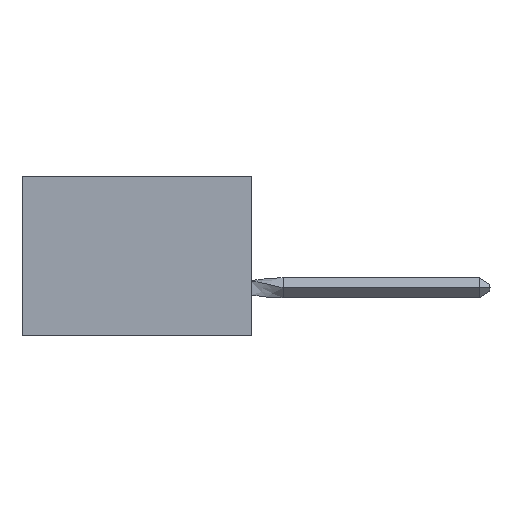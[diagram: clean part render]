
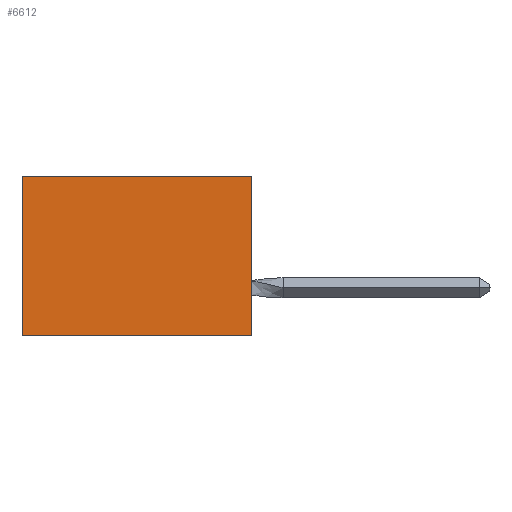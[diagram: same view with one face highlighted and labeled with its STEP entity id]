
A CAD part, left-side view. The second image highlights one B-rep face of the part: STEP entity #6612.
In plain terms, the highlighted planar face has unit normal (-1, 0, 0).
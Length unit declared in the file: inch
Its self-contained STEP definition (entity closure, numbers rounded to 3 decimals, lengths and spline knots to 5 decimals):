
#203 = VECTOR ( 'NONE', #4181, 39.37008 ) ;
#542 = PLANE ( 'NONE',  #6799 ) ;
#1179 = VECTOR ( 'NONE', #8908, 39.37008 ) ;
#1375 = EDGE_LOOP ( 'NONE', ( #3609, #6188, #13328, #8357 ) ) ;
#1581 = CARTESIAN_POINT ( 'NONE',  ( 0.305, 0., -0.5 ) ) ;
#2158 = VERTEX_POINT ( 'NONE', #9919 ) ;
#2236 = VECTOR ( 'NONE', #9385, 39.37008 ) ;
#2785 = LINE ( 'NONE', #3702, #1179 ) ;
#2906 = LINE ( 'NONE', #4169, #2236 ) ;
#3089 = EDGE_CURVE ( 'NONE', #11023, #5474, #4993, .T. ) ;
#3609 = ORIENTED_EDGE ( 'NONE', *, *, #3977, .T. ) ;
#3682 = VECTOR ( 'NONE', #5575, 39.37008 ) ;
#3702 = CARTESIAN_POINT ( 'NONE',  ( 0.305, 0., 0. ) ) ;
#3977 = EDGE_CURVE ( 'NONE', #4420, #5474, #2906, .T. ) ;
#4169 = CARTESIAN_POINT ( 'NONE',  ( 0.305, 0.72, -0.5 ) ) ;
#4181 = DIRECTION ( 'NONE',  ( 0., 0., -1. ) ) ;
#4420 = VERTEX_POINT ( 'NONE', #10097 ) ;
#4819 = CARTESIAN_POINT ( 'NONE',  ( 0.305, 0., -0.5 ) ) ;
#4993 = LINE ( 'NONE', #10900, #3682 ) ;
#5042 = LINE ( 'NONE', #6329, #203 ) ;
#5474 = VERTEX_POINT ( 'NONE', #9272 ) ;
#5575 = DIRECTION ( 'NONE',  ( 0., 1., 0. ) ) ;
#6188 = ORIENTED_EDGE ( 'NONE', *, *, #3089, .F. ) ;
#6329 = CARTESIAN_POINT ( 'NONE',  ( 0.305, 0., -0.5 ) ) ;
#6612 = ADVANCED_FACE ( 'NONE', ( #12979 ), #542, .F. ) ;
#6782 = EDGE_CURVE ( 'NONE', #2158, #11023, #5042, .T. ) ;
#6799 = AXIS2_PLACEMENT_3D ( 'NONE', #1581, #8815, #10877 ) ;
#8357 = ORIENTED_EDGE ( 'NONE', *, *, #12639, .T. ) ;
#8815 = DIRECTION ( 'NONE',  ( 1., 0., 0. ) ) ;
#8908 = DIRECTION ( 'NONE',  ( 0., 1., 0. ) ) ;
#9272 = CARTESIAN_POINT ( 'NONE',  ( 0.305, 0.72, -0.5 ) ) ;
#9385 = DIRECTION ( 'NONE',  ( 0., 0., -1. ) ) ;
#9919 = CARTESIAN_POINT ( 'NONE',  ( 0.305, 0., 0. ) ) ;
#10097 = CARTESIAN_POINT ( 'NONE',  ( 0.305, 0.72, 0. ) ) ;
#10877 = DIRECTION ( 'NONE',  ( 0., 0., -1. ) ) ;
#10900 = CARTESIAN_POINT ( 'NONE',  ( 0.305, 0., -0.5 ) ) ;
#11023 = VERTEX_POINT ( 'NONE', #4819 ) ;
#12639 = EDGE_CURVE ( 'NONE', #2158, #4420, #2785, .T. ) ;
#12979 = FACE_OUTER_BOUND ( 'NONE', #1375, .T. ) ;
#13328 = ORIENTED_EDGE ( 'NONE', *, *, #6782, .F. ) ;
